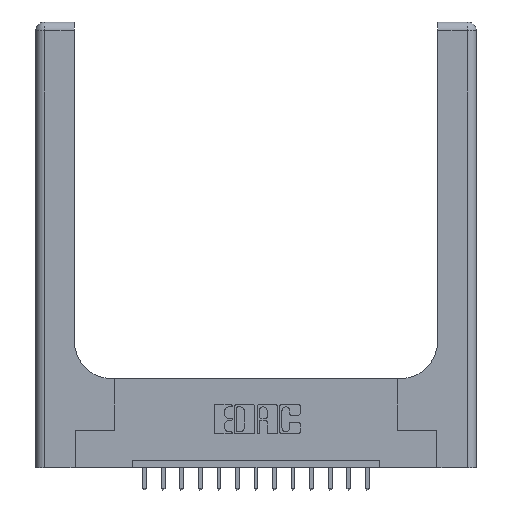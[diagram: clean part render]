
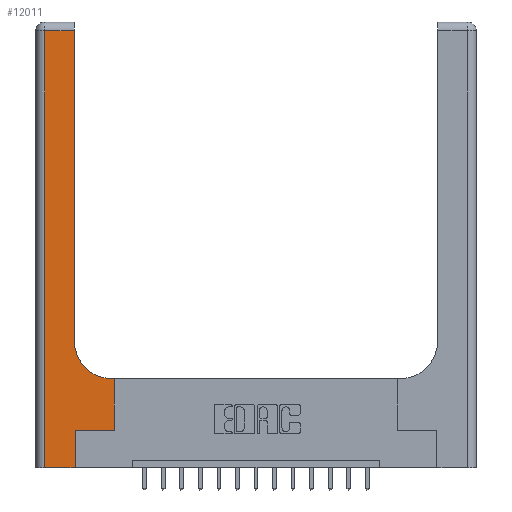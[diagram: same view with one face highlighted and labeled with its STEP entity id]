
A CAD part, top view. The second image highlights one B-rep face of the part: STEP entity #12011.
In plain terms, the highlighted planar face has unit normal (0, 0, 1).
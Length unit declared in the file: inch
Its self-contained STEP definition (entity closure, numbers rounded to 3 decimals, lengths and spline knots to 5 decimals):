
#213 = VERTEX_POINT ( 'NONE', #17573 ) ;
#529 = LINE ( 'NONE', #4607, #12066 ) ;
#619 = VECTOR ( 'NONE', #8979, 39.37008 ) ;
#1146 = DIRECTION ( 'NONE',  ( 0., 1., 0. ) ) ;
#1202 = VERTEX_POINT ( 'NONE', #1609 ) ;
#1391 = CARTESIAN_POINT ( 'NONE',  ( 0.265, 0.25, 0.37 ) ) ;
#1482 = LINE ( 'NONE', #1391, #3447 ) ;
#1484 = VECTOR ( 'NONE', #10931, 39.37008 ) ;
#1609 = CARTESIAN_POINT ( 'NONE',  ( 0.528, 0.6, 0.37 ) ) ;
#1688 = LINE ( 'NONE', #5973, #2017 ) ;
#1766 = VECTOR ( 'NONE', #5999, 39.37008 ) ;
#2017 = VECTOR ( 'NONE', #4624, 39.37008 ) ;
#2038 = LINE ( 'NONE', #9876, #7078 ) ;
#2270 = VERTEX_POINT ( 'NONE', #12407 ) ;
#2769 = CIRCLE ( 'NONE', #13311, 0.25 ) ;
#3301 = DIRECTION ( 'NONE',  ( 1., 0., 0. ) ) ;
#3337 = EDGE_CURVE ( 'NONE', #1202, #8458, #12512, .T. ) ;
#3447 = VECTOR ( 'NONE', #7899, 39.37008 ) ;
#3489 = DIRECTION ( 'NONE',  ( -1., 0., 0. ) ) ;
#3610 = CARTESIAN_POINT ( 'NONE',  ( 0.265, 0., 0.37 ) ) ;
#3633 = LINE ( 'NONE', #17266, #15150 ) ;
#4482 = CARTESIAN_POINT ( 'NONE',  ( 0.26, 0.6, 0.37 ) ) ;
#4607 = CARTESIAN_POINT ( 'NONE',  ( 0.265, 0., 0.37 ) ) ;
#4624 = DIRECTION ( 'NONE',  ( -1., 0., 0. ) ) ;
#5355 = EDGE_CURVE ( 'NONE', #8458, #13473, #2769, .T. ) ;
#5676 = VERTEX_POINT ( 'NONE', #10891 ) ;
#5869 = EDGE_CURVE ( 'NONE', #12785, #16279, #2038, .T. ) ;
#5973 = CARTESIAN_POINT ( 'NONE',  ( 0., 2.94, 0.37 ) ) ;
#5999 = DIRECTION ( 'NONE',  ( 0., -1., 0. ) ) ;
#6039 = EDGE_CURVE ( 'NONE', #8608, #1202, #3633, .T. ) ;
#7078 = VECTOR ( 'NONE', #12915, 39.37008 ) ;
#7229 = ORIENTED_EDGE ( 'NONE', *, *, #10449, .T. ) ;
#7314 = LINE ( 'NONE', #7577, #1766 ) ;
#7577 = CARTESIAN_POINT ( 'NONE',  ( 0.06, 3., 0.37 ) ) ;
#7899 = DIRECTION ( 'NONE',  ( 1., 0., 0. ) ) ;
#8190 = ORIENTED_EDGE ( 'NONE', *, *, #11910, .T. ) ;
#8458 = VERTEX_POINT ( 'NONE', #14527 ) ;
#8608 = VERTEX_POINT ( 'NONE', #13828 ) ;
#8685 = CARTESIAN_POINT ( 'NONE',  ( 0.06, 0., 0.37 ) ) ;
#8979 = DIRECTION ( 'NONE',  ( 0., 1., 0. ) ) ;
#9132 = ORIENTED_EDGE ( 'NONE', *, *, #3337, .T. ) ;
#9697 = ORIENTED_EDGE ( 'NONE', *, *, #5869, .T. ) ;
#9876 = CARTESIAN_POINT ( 'NONE',  ( 0., 0., 0.37 ) ) ;
#10449 = EDGE_CURVE ( 'NONE', #2270, #5676, #1688, .T. ) ;
#10488 = LINE ( 'NONE', #15641, #619 ) ;
#10891 = CARTESIAN_POINT ( 'NONE',  ( 0.06, 2.94, 0.37 ) ) ;
#10931 = DIRECTION ( 'NONE',  ( -1., 0., 0. ) ) ;
#10988 = EDGE_CURVE ( 'NONE', #13473, #2270, #10488, .T. ) ;
#11135 = DIRECTION ( 'NONE',  ( 0., 1., 0. ) ) ;
#11187 = EDGE_CURVE ( 'NONE', #213, #8608, #1482, .T. ) ;
#11910 = EDGE_CURVE ( 'NONE', #5676, #12785, #7314, .T. ) ;
#12011 = ADVANCED_FACE ( 'NONE', ( #17031 ), #15687, .F. ) ;
#12066 = VECTOR ( 'NONE', #11135, 39.37008 ) ;
#12407 = CARTESIAN_POINT ( 'NONE',  ( 0.26, 2.94, 0.37 ) ) ;
#12512 = LINE ( 'NONE', #4482, #1484 ) ;
#12680 = ORIENTED_EDGE ( 'NONE', *, *, #6039, .T. ) ;
#12785 = VERTEX_POINT ( 'NONE', #8685 ) ;
#12844 = DIRECTION ( 'NONE',  ( 0., 0., -1. ) ) ;
#12915 = DIRECTION ( 'NONE',  ( 1., 0., 0. ) ) ;
#13311 = AXIS2_PLACEMENT_3D ( 'NONE', #14172, #12844, #3301 ) ;
#13473 = VERTEX_POINT ( 'NONE', #17473 ) ;
#13495 = ORIENTED_EDGE ( 'NONE', *, *, #11187, .T. ) ;
#13828 = CARTESIAN_POINT ( 'NONE',  ( 0.528, 0.25, 0.37 ) ) ;
#14172 = CARTESIAN_POINT ( 'NONE',  ( 0.51, 0.85, 0.37 ) ) ;
#14224 = ORIENTED_EDGE ( 'NONE', *, *, #5355, .T. ) ;
#14527 = CARTESIAN_POINT ( 'NONE',  ( 0.51, 0.6, 0.37 ) ) ;
#15150 = VECTOR ( 'NONE', #1146, 39.37008 ) ;
#15243 = EDGE_CURVE ( 'NONE', #16279, #213, #529, .T. ) ;
#15376 = AXIS2_PLACEMENT_3D ( 'NONE', #16861, #17118, #3489 ) ;
#15641 = CARTESIAN_POINT ( 'NONE',  ( 0.26, 3., 0.37 ) ) ;
#15687 = PLANE ( 'NONE',  #15376 ) ;
#16279 = VERTEX_POINT ( 'NONE', #3610 ) ;
#16584 = ORIENTED_EDGE ( 'NONE', *, *, #10988, .T. ) ;
#16861 = CARTESIAN_POINT ( 'NONE',  ( 0., 3., 0.37 ) ) ;
#17031 = FACE_OUTER_BOUND ( 'NONE', #17105, .T. ) ;
#17105 = EDGE_LOOP ( 'NONE', ( #16584, #7229, #8190, #9697, #17120, #13495, #12680, #9132, #14224 ) ) ;
#17118 = DIRECTION ( 'NONE',  ( 0., 0., -1. ) ) ;
#17120 = ORIENTED_EDGE ( 'NONE', *, *, #15243, .T. ) ;
#17266 = CARTESIAN_POINT ( 'NONE',  ( 0.528, 0.25, 0.37 ) ) ;
#17473 = CARTESIAN_POINT ( 'NONE',  ( 0.26, 0.85, 0.37 ) ) ;
#17573 = CARTESIAN_POINT ( 'NONE',  ( 0.265, 0.25, 0.37 ) ) ;
